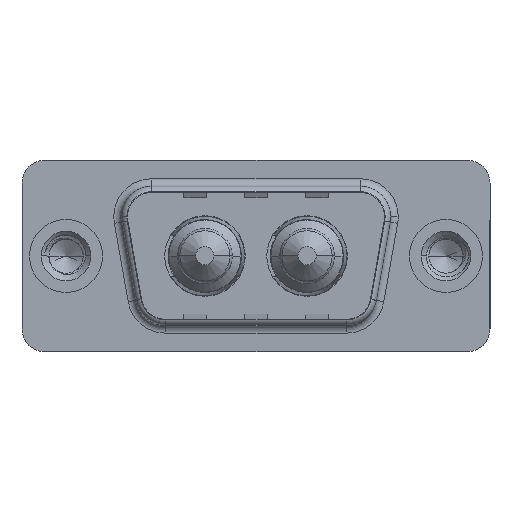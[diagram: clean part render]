
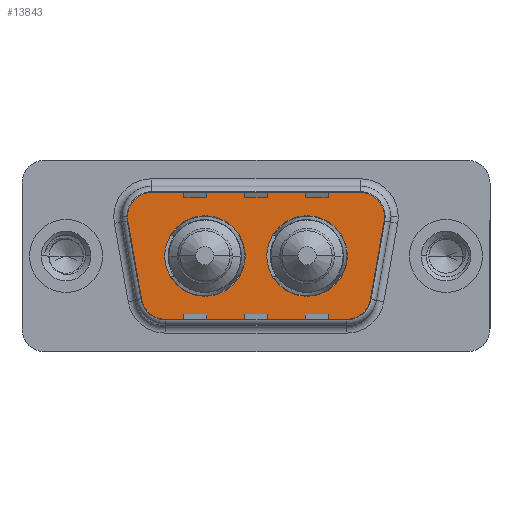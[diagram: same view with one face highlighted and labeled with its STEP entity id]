
A CAD part, top view. The second image highlights one B-rep face of the part: STEP entity #13843.
In plain terms, the highlighted planar face has unit normal (0, 0, 1).
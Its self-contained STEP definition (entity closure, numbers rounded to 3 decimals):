
#208 = ORIENTED_EDGE ( 'NONE', *, *, #2509, .T. ) ;
#266 = CIRCLE ( 'NONE', #2061, 2.65 ) ;
#598 = CARTESIAN_POINT ( 'NONE',  ( 4.489, -3.247, 0. ) ) ;
#1232 = CIRCLE ( 'NONE', #2856, 2.65 ) ;
#1567 = PLANE ( 'NONE',  #15505 ) ;
#1762 = CARTESIAN_POINT ( 'NONE',  ( 19.564, 4.9, 0. ) ) ;
#1838 = EDGE_CURVE ( 'NONE', #11473, #11010, #9193, .T. ) ;
#2011 = VERTEX_POINT ( 'NONE', #10269 ) ;
#2061 = AXIS2_PLACEMENT_3D ( 'NONE', #10674, #13126, #7536 ) ;
#2079 = ORIENTED_EDGE ( 'NONE', *, *, #7546, .T. ) ;
#2509 = EDGE_CURVE ( 'NONE', #3047, #14332, #14840, .T. ) ;
#2856 = AXIS2_PLACEMENT_3D ( 'NONE', #12082, #10614, #4074 ) ;
#2924 = CARTESIAN_POINT ( 'NONE',  ( 21.534, 2.553, 0. ) ) ;
#2978 = ORIENTED_EDGE ( 'NONE', *, *, #12343, .T. ) ;
#3047 = VERTEX_POINT ( 'NONE', #15349 ) ;
#3110 = DIRECTION ( 'NONE',  ( 0., 0., 1. ) ) ;
#3171 = VERTEX_POINT ( 'NONE', #598 ) ;
#3490 = CARTESIAN_POINT ( 'NONE',  ( 3.466, 2.553, 0. ) ) ;
#3653 = CARTESIAN_POINT ( 'NONE',  ( 6.459, -2.9, 0. ) ) ;
#3795 = DIRECTION ( 'NONE',  ( 0., 0., 1. ) ) ;
#4057 = CIRCLE ( 'NONE', #12963, 2. ) ;
#4073 = VERTEX_POINT ( 'NONE', #1762 ) ;
#4074 = DIRECTION ( 'NONE',  ( 1., 0., 0. ) ) ;
#4309 = LINE ( 'NONE', #7610, #13246 ) ;
#4447 = EDGE_CURVE ( 'NONE', #2011, #8535, #8403, .T. ) ;
#4681 = CIRCLE ( 'NONE', #8162, 2. ) ;
#4687 = AXIS2_PLACEMENT_3D ( 'NONE', #14703, #7065, #16008 ) ;
#4796 = ORIENTED_EDGE ( 'NONE', *, *, #15391, .T. ) ;
#4947 = EDGE_CURVE ( 'NONE', #10210, #11836, #266, .T. ) ;
#4951 = DIRECTION ( 'NONE',  ( -1., 0., 0. ) ) ;
#5066 = DIRECTION ( 'NONE',  ( -1., 0., 0. ) ) ;
#5260 = CARTESIAN_POINT ( 'NONE',  ( 3.466, 2.553, 0. ) ) ;
#5268 = DIRECTION ( 'NONE',  ( 0.174, 0.985, 0. ) ) ;
#5269 = CIRCLE ( 'NONE', #4687, 2.65 ) ;
#5371 = DIRECTION ( 'NONE',  ( 1., 0., 0. ) ) ;
#5392 = AXIS2_PLACEMENT_3D ( 'NONE', #7540, #16513, #8762 ) ;
#5424 = ORIENTED_EDGE ( 'NONE', *, *, #4947, .F. ) ;
#5546 = CARTESIAN_POINT ( 'NONE',  ( 5.436, 2.9, 0. ) ) ;
#5627 = VECTOR ( 'NONE', #14149, 1000. ) ;
#5778 = ORIENTED_EDGE ( 'NONE', *, *, #1838, .F. ) ;
#5823 = EDGE_CURVE ( 'NONE', #11836, #10210, #1232, .T. ) ;
#5963 = EDGE_LOOP ( 'NONE', ( #5424, #8025 ) ) ;
#6507 = EDGE_CURVE ( 'NONE', #9924, #12753, #10105, .T. ) ;
#6547 = DIRECTION ( 'NONE',  ( 1., 0., 0. ) ) ;
#6594 = LINE ( 'NONE', #2924, #15985 ) ;
#6727 = DIRECTION ( 'NONE',  ( 1., 0., 0. ) ) ;
#6830 = DIRECTION ( 'NONE',  ( 1., 0., 0. ) ) ;
#6858 = FACE_BOUND ( 'NONE', #7360, .T. ) ;
#7065 = DIRECTION ( 'NONE',  ( 0., 0., 1. ) ) ;
#7360 = EDGE_LOOP ( 'NONE', ( #5778, #14134 ) ) ;
#7440 = CARTESIAN_POINT ( 'NONE',  ( 19.564, 2.9, 0. ) ) ;
#7536 = DIRECTION ( 'NONE',  ( 1., 0., 0. ) ) ;
#7540 = CARTESIAN_POINT ( 'NONE',  ( 18.541, -2.9, 0. ) ) ;
#7546 = EDGE_CURVE ( 'NONE', #9531, #3047, #6594, .T. ) ;
#7581 = ORIENTED_EDGE ( 'NONE', *, *, #6507, .T. ) ;
#7610 = CARTESIAN_POINT ( 'NONE',  ( 5.436, 4.9, 0. ) ) ;
#7764 = CARTESIAN_POINT ( 'NONE',  ( 13.21, 0., 0. ) ) ;
#8025 = ORIENTED_EDGE ( 'NONE', *, *, #5823, .F. ) ;
#8162 = AXIS2_PLACEMENT_3D ( 'NONE', #7440, #16407, #8654 ) ;
#8390 = EDGE_LOOP ( 'NONE', ( #10660, #2079, #208, #2978, #14603, #7581, #4796, #10234, #14731 ) ) ;
#8403 = LINE ( 'NONE', #9084, #14844 ) ;
#8535 = VERTEX_POINT ( 'NONE', #10887 ) ;
#8654 = DIRECTION ( 'NONE',  ( -1., 0., 0. ) ) ;
#8670 = EDGE_CURVE ( 'NONE', #8535, #9531, #9272, .T. ) ;
#8762 = DIRECTION ( 'NONE',  ( 1., 0., 0. ) ) ;
#9084 = CARTESIAN_POINT ( 'NONE',  ( 6.459, -4.9, 0. ) ) ;
#9193 = CIRCLE ( 'NONE', #10352, 2.65 ) ;
#9272 = CIRCLE ( 'NONE', #5392, 2. ) ;
#9531 = VERTEX_POINT ( 'NONE', #12873 ) ;
#9585 = CARTESIAN_POINT ( 'NONE',  ( 5.436, 4.9, 0. ) ) ;
#9910 = DIRECTION ( 'NONE',  ( -1., 0., 0. ) ) ;
#9924 = VERTEX_POINT ( 'NONE', #9585 ) ;
#10105 = CIRCLE ( 'NONE', #15903, 2. ) ;
#10136 = FACE_OUTER_BOUND ( 'NONE', #8390, .T. ) ;
#10210 = VERTEX_POINT ( 'NONE', #14689 ) ;
#10234 = ORIENTED_EDGE ( 'NONE', *, *, #12829, .T. ) ;
#10269 = CARTESIAN_POINT ( 'NONE',  ( 6.459, -4.9, 0. ) ) ;
#10352 = AXIS2_PLACEMENT_3D ( 'NONE', #11019, #3110, #5371 ) ;
#10436 = CARTESIAN_POINT ( 'NONE',  ( 19.564, 2.9, 0. ) ) ;
#10468 = CARTESIAN_POINT ( 'NONE',  ( 21.564, 2.9, 0. ) ) ;
#10614 = DIRECTION ( 'NONE',  ( 0., 0., 1. ) ) ;
#10660 = ORIENTED_EDGE ( 'NONE', *, *, #8670, .T. ) ;
#10674 = CARTESIAN_POINT ( 'NONE',  ( 15.86, 0., 0. ) ) ;
#10887 = CARTESIAN_POINT ( 'NONE',  ( 18.541, -4.9, 0. ) ) ;
#10907 = CARTESIAN_POINT ( 'NONE',  ( 11.79, 0., 0. ) ) ;
#11010 = VERTEX_POINT ( 'NONE', #12770 ) ;
#11019 = CARTESIAN_POINT ( 'NONE',  ( 9.14, 0., 0. ) ) ;
#11473 = VERTEX_POINT ( 'NONE', #10907 ) ;
#11671 = CARTESIAN_POINT ( 'NONE',  ( 18.541, -2.9, 0. ) ) ;
#11739 = EDGE_CURVE ( 'NONE', #4073, #9924, #4309, .T. ) ;
#11836 = VERTEX_POINT ( 'NONE', #7764 ) ;
#12082 = CARTESIAN_POINT ( 'NONE',  ( 15.86, 0., 0. ) ) ;
#12237 = DIRECTION ( 'NONE',  ( 0., 0., 1. ) ) ;
#12343 = EDGE_CURVE ( 'NONE', #14332, #4073, #4681, .T. ) ;
#12513 = DIRECTION ( 'NONE',  ( 0., 0., 1. ) ) ;
#12753 = VERTEX_POINT ( 'NONE', #3490 ) ;
#12770 = CARTESIAN_POINT ( 'NONE',  ( 6.49, 0., 0. ) ) ;
#12829 = EDGE_CURVE ( 'NONE', #3171, #2011, #4057, .T. ) ;
#12873 = CARTESIAN_POINT ( 'NONE',  ( 20.511, -3.247, 0. ) ) ;
#12963 = AXIS2_PLACEMENT_3D ( 'NONE', #3653, #12513, #4951 ) ;
#13126 = DIRECTION ( 'NONE',  ( 0., 0., 1. ) ) ;
#13246 = VECTOR ( 'NONE', #5066, 1000. ) ;
#13357 = EDGE_CURVE ( 'NONE', #11010, #11473, #5269, .T. ) ;
#13580 = FACE_BOUND ( 'NONE', #5963, .T. ) ;
#13843 = ADVANCED_FACE ( 'NONE', ( #13580, #6858, #10136 ), #1567, .T. ) ;
#14077 = AXIS2_PLACEMENT_3D ( 'NONE', #10436, #12237, #9910 ) ;
#14134 = ORIENTED_EDGE ( 'NONE', *, *, #13357, .F. ) ;
#14149 = DIRECTION ( 'NONE',  ( 0.174, -0.985, 0. ) ) ;
#14332 = VERTEX_POINT ( 'NONE', #10468 ) ;
#14351 = DIRECTION ( 'NONE',  ( 0., 0., 1. ) ) ;
#14603 = ORIENTED_EDGE ( 'NONE', *, *, #11739, .T. ) ;
#14689 = CARTESIAN_POINT ( 'NONE',  ( 18.51, 0., 0. ) ) ;
#14703 = CARTESIAN_POINT ( 'NONE',  ( 9.14, 0., 0. ) ) ;
#14731 = ORIENTED_EDGE ( 'NONE', *, *, #4447, .T. ) ;
#14840 = CIRCLE ( 'NONE', #14077, 2. ) ;
#14844 = VECTOR ( 'NONE', #6547, 1000. ) ;
#15349 = CARTESIAN_POINT ( 'NONE',  ( 21.534, 2.553, 0. ) ) ;
#15391 = EDGE_CURVE ( 'NONE', #12753, #3171, #15409, .T. ) ;
#15409 = LINE ( 'NONE', #5260, #5627 ) ;
#15505 = AXIS2_PLACEMENT_3D ( 'NONE', #11671, #14351, #6727 ) ;
#15903 = AXIS2_PLACEMENT_3D ( 'NONE', #5546, #3795, #6830 ) ;
#15985 = VECTOR ( 'NONE', #5268, 1000. ) ;
#16008 = DIRECTION ( 'NONE',  ( 1., 0., 0. ) ) ;
#16407 = DIRECTION ( 'NONE',  ( 0., 0., 1. ) ) ;
#16513 = DIRECTION ( 'NONE',  ( 0., 0., 1. ) ) ;
